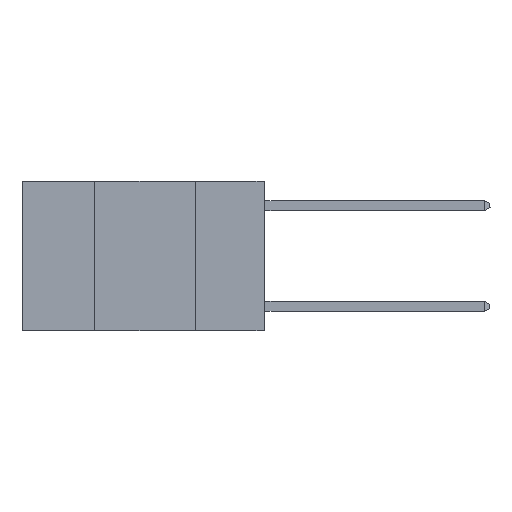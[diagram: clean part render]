
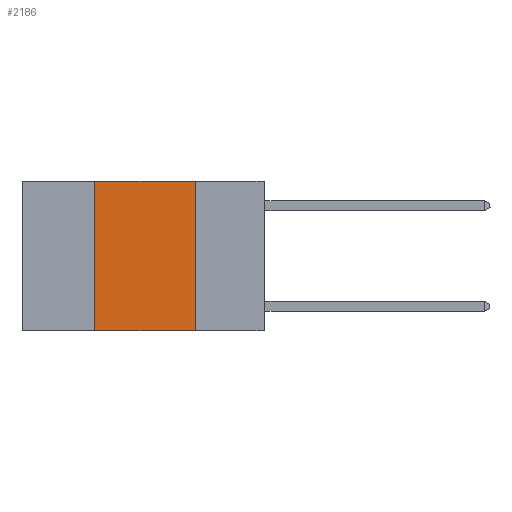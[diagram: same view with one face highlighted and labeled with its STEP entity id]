
A CAD part, left-side view. The second image highlights one B-rep face of the part: STEP entity #2186.
In plain terms, the highlighted planar face has unit normal (-1, 0, 0).
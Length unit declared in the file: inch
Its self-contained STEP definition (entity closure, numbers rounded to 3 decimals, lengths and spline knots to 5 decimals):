
#210 = EDGE_LOOP ( 'NONE', ( #2365, #8795, #7161, #4333 ) ) ;
#220 = AXIS2_PLACEMENT_3D ( 'NONE', #8084, #8539, #6264 ) ;
#468 = VECTOR ( 'NONE', #2526, 39.37008 ) ;
#837 = FACE_OUTER_BOUND ( 'NONE', #210, .T. ) ;
#1547 = CARTESIAN_POINT ( 'NONE',  ( 0., 0.6, -0.37 ) ) ;
#1747 = VERTEX_POINT ( 'NONE', #3441 ) ;
#2186 = ADVANCED_FACE ( 'NONE', ( #837 ), #6674, .F. ) ;
#2225 = VECTOR ( 'NONE', #6736, 39.37008 ) ;
#2352 = CARTESIAN_POINT ( 'NONE',  ( 0., 0.42, -0.37 ) ) ;
#2365 = ORIENTED_EDGE ( 'NONE', *, *, #3201, .F. ) ;
#2408 = VERTEX_POINT ( 'NONE', #6364 ) ;
#2526 = DIRECTION ( 'NONE',  ( 0., -1., 0. ) ) ;
#2589 = VECTOR ( 'NONE', #5033, 39.37008 ) ;
#3201 = EDGE_CURVE ( 'NONE', #5615, #2408, #10010, .T. ) ;
#3236 = EDGE_CURVE ( 'NONE', #5548, #1747, #9278, .T. ) ;
#3441 = CARTESIAN_POINT ( 'NONE',  ( 0., 0.42, 0. ) ) ;
#4148 = CARTESIAN_POINT ( 'NONE',  ( 0., 0.42, 0. ) ) ;
#4333 = ORIENTED_EDGE ( 'NONE', *, *, #6784, .T. ) ;
#5033 = DIRECTION ( 'NONE',  ( 0., 0., 1. ) ) ;
#5548 = VERTEX_POINT ( 'NONE', #2352 ) ;
#5615 = VERTEX_POINT ( 'NONE', #9135 ) ;
#5872 = CARTESIAN_POINT ( 'NONE',  ( 0., 0.6, 0. ) ) ;
#6264 = DIRECTION ( 'NONE',  ( 0., 0., -1. ) ) ;
#6364 = CARTESIAN_POINT ( 'NONE',  ( 0., 0.17, -0.37 ) ) ;
#6674 = PLANE ( 'NONE',  #220 ) ;
#6736 = DIRECTION ( 'NONE',  ( 0., -1., 0. ) ) ;
#6784 = EDGE_CURVE ( 'NONE', #5548, #2408, #7513, .T. ) ;
#6980 = EDGE_CURVE ( 'NONE', #1747, #5615, #8974, .T. ) ;
#7161 = ORIENTED_EDGE ( 'NONE', *, *, #3236, .F. ) ;
#7513 = LINE ( 'NONE', #1547, #468 ) ;
#7686 = VECTOR ( 'NONE', #8178, 39.37008 ) ;
#8084 = CARTESIAN_POINT ( 'NONE',  ( 0., 0.6, 0. ) ) ;
#8178 = DIRECTION ( 'NONE',  ( 0., 0., -1. ) ) ;
#8539 = DIRECTION ( 'NONE',  ( 1., 0., 0. ) ) ;
#8795 = ORIENTED_EDGE ( 'NONE', *, *, #6980, .F. ) ;
#8974 = LINE ( 'NONE', #5872, #2225 ) ;
#9135 = CARTESIAN_POINT ( 'NONE',  ( 0., 0.17, 0. ) ) ;
#9278 = LINE ( 'NONE', #4148, #2589 ) ;
#10010 = LINE ( 'NONE', #10538, #7686 ) ;
#10538 = CARTESIAN_POINT ( 'NONE',  ( 0., 0.17, 0. ) ) ;
